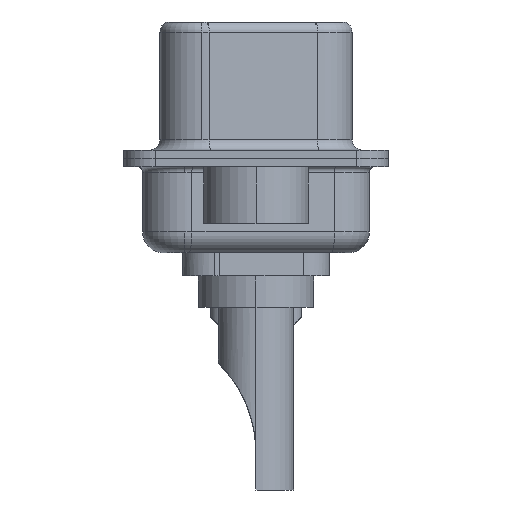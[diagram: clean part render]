
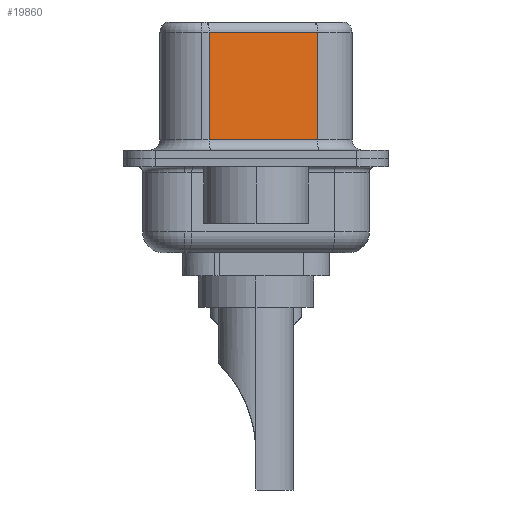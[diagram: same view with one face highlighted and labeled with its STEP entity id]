
A CAD part, left-side view. The second image highlights one B-rep face of the part: STEP entity #19860.
In plain terms, the highlighted planar face has unit normal (-0.985, -0.174, 0).
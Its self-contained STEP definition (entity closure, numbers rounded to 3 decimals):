
#253 = CARTESIAN_POINT ( 'NONE',  ( 4.58, -2.927, 6.52 ) ) ;
#1775 = EDGE_LOOP ( 'NONE', ( #24546, #7396, #3868, #24058 ) ) ;
#3868 = ORIENTED_EDGE ( 'NONE', *, *, #12196, .T. ) ;
#6146 = DIRECTION ( 'NONE',  ( 0., 0., -1. ) ) ;
#6256 = DIRECTION ( 'NONE',  ( -0.174, 0.985, 0. ) ) ;
#6436 = EDGE_CURVE ( 'NONE', #24919, #11467, #7888, .T. ) ;
#6729 = CARTESIAN_POINT ( 'NONE',  ( 4.58, -2.927, 0.9 ) ) ;
#7396 = ORIENTED_EDGE ( 'NONE', *, *, #8401, .T. ) ;
#7888 = LINE ( 'NONE', #16064, #23097 ) ;
#8371 = FACE_OUTER_BOUND ( 'NONE', #1775, .T. ) ;
#8401 = EDGE_CURVE ( 'NONE', #24919, #13580, #11784, .T. ) ;
#8408 = LINE ( 'NONE', #6729, #18320 ) ;
#9310 = VERTEX_POINT ( 'NONE', #17955 ) ;
#9445 = CARTESIAN_POINT ( 'NONE',  ( 4.58, -2.927, 6.02 ) ) ;
#9913 = AXIS2_PLACEMENT_3D ( 'NONE', #253, #18156, #6256 ) ;
#11467 = VERTEX_POINT ( 'NONE', #15231 ) ;
#11784 = LINE ( 'NONE', #9445, #17031 ) ;
#12196 = EDGE_CURVE ( 'NONE', #13580, #9310, #20331, .T. ) ;
#13076 = CARTESIAN_POINT ( 'NONE',  ( 4.58, -2.927, 6.02 ) ) ;
#13580 = VERTEX_POINT ( 'NONE', #13829 ) ;
#13829 = CARTESIAN_POINT ( 'NONE',  ( 3.67, 2.233, 6.02 ) ) ;
#14457 = VECTOR ( 'NONE', #25677, 1000. ) ;
#15231 = CARTESIAN_POINT ( 'NONE',  ( 4.58, -2.927, 0.9 ) ) ;
#16064 = CARTESIAN_POINT ( 'NONE',  ( 4.58, -2.927, 6.52 ) ) ;
#16166 = PLANE ( 'NONE',  #9913 ) ;
#16629 = DIRECTION ( 'NONE',  ( 0.174, -0.985, 0. ) ) ;
#17031 = VECTOR ( 'NONE', #25268, 1000. ) ;
#17955 = CARTESIAN_POINT ( 'NONE',  ( 3.67, 2.233, 0.9 ) ) ;
#18156 = DIRECTION ( 'NONE',  ( 0.985, 0.174, 0. ) ) ;
#18320 = VECTOR ( 'NONE', #16629, 1000. ) ;
#19860 = ADVANCED_FACE ( 'NONE', ( #8371 ), #16166, .F. ) ;
#20331 = LINE ( 'NONE', #25754, #14457 ) ;
#23097 = VECTOR ( 'NONE', #6146, 1000. ) ;
#24058 = ORIENTED_EDGE ( 'NONE', *, *, #24904, .T. ) ;
#24546 = ORIENTED_EDGE ( 'NONE', *, *, #6436, .F. ) ;
#24904 = EDGE_CURVE ( 'NONE', #9310, #11467, #8408, .T. ) ;
#24919 = VERTEX_POINT ( 'NONE', #13076 ) ;
#25268 = DIRECTION ( 'NONE',  ( -0.174, 0.985, 0. ) ) ;
#25677 = DIRECTION ( 'NONE',  ( 0., 0., -1. ) ) ;
#25754 = CARTESIAN_POINT ( 'NONE',  ( 3.67, 2.233, 6.52 ) ) ;
